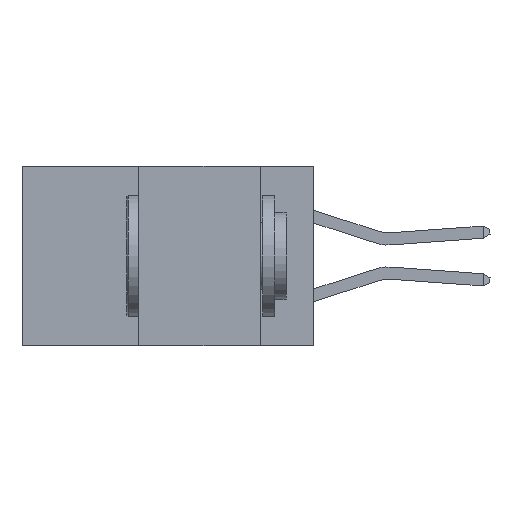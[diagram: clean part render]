
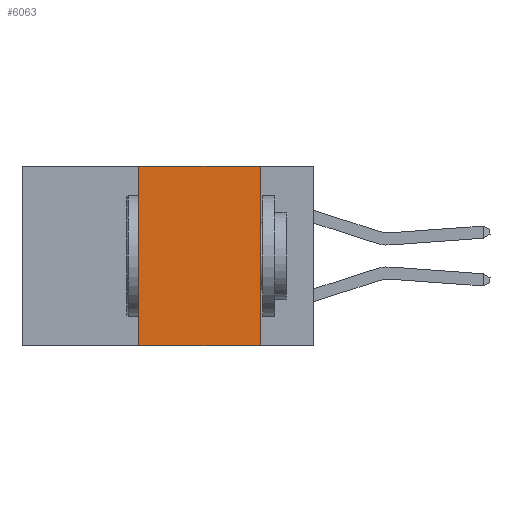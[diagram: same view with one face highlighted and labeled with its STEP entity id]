
A CAD part, left-side view. The second image highlights one B-rep face of the part: STEP entity #6063.
In plain terms, the highlighted planar face has unit normal (-1, 0, 0).
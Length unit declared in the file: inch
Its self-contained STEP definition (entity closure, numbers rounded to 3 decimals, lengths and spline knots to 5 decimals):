
#858 = AXIS2_PLACEMENT_3D ( 'NONE', #20803, #15157, #6983 ) ;
#1157 = VECTOR ( 'NONE', #2680, 39.37008 ) ;
#2680 = DIRECTION ( 'NONE',  ( 0., -1., 0. ) ) ;
#4364 = EDGE_CURVE ( 'NONE', #21309, #8622, #9887, .T. ) ;
#4973 = EDGE_LOOP ( 'NONE', ( #7449, #23508, #30149, #10833 ) ) ;
#5776 = VECTOR ( 'NONE', #22910, 39.37008 ) ;
#6063 = ADVANCED_FACE ( 'NONE', ( #34013 ), #12747, .F. ) ;
#6983 = DIRECTION ( 'NONE',  ( 0., 0., -1. ) ) ;
#6994 = VERTEX_POINT ( 'NONE', #29694 ) ;
#7449 = ORIENTED_EDGE ( 'NONE', *, *, #15761, .F. ) ;
#8044 = EDGE_CURVE ( 'NONE', #6994, #9968, #10895, .T. ) ;
#8622 = VERTEX_POINT ( 'NONE', #16449 ) ;
#9887 = LINE ( 'NONE', #34178, #32838 ) ;
#9968 = VERTEX_POINT ( 'NONE', #29895 ) ;
#10833 = ORIENTED_EDGE ( 'NONE', *, *, #8044, .T. ) ;
#10847 = DIRECTION ( 'NONE',  ( 0., 0., -1. ) ) ;
#10895 = LINE ( 'NONE', #16295, #1157 ) ;
#11619 = CARTESIAN_POINT ( 'NONE',  ( 0., 0.36, 0. ) ) ;
#12086 = LINE ( 'NONE', #20289, #5776 ) ;
#12123 = LINE ( 'NONE', #16080, #15553 ) ;
#12747 = PLANE ( 'NONE',  #858 ) ;
#15157 = DIRECTION ( 'NONE',  ( 1., 0., 0. ) ) ;
#15553 = VECTOR ( 'NONE', #10847, 39.37008 ) ;
#15761 = EDGE_CURVE ( 'NONE', #8622, #9968, #12123, .T. ) ;
#16080 = CARTESIAN_POINT ( 'NONE',  ( 0., 0.11, 0. ) ) ;
#16295 = CARTESIAN_POINT ( 'NONE',  ( 0., 0.6, -0.37 ) ) ;
#16449 = CARTESIAN_POINT ( 'NONE',  ( 0., 0.11, 0. ) ) ;
#20289 = CARTESIAN_POINT ( 'NONE',  ( 0., 0.36, 0. ) ) ;
#20803 = CARTESIAN_POINT ( 'NONE',  ( 0., 0.6, 0. ) ) ;
#21309 = VERTEX_POINT ( 'NONE', #11619 ) ;
#22910 = DIRECTION ( 'NONE',  ( 0., 0., 1. ) ) ;
#23508 = ORIENTED_EDGE ( 'NONE', *, *, #4364, .F. ) ;
#25860 = DIRECTION ( 'NONE',  ( 0., -1., 0. ) ) ;
#29694 = CARTESIAN_POINT ( 'NONE',  ( 0., 0.36, -0.37 ) ) ;
#29895 = CARTESIAN_POINT ( 'NONE',  ( 0., 0.11, -0.37 ) ) ;
#30149 = ORIENTED_EDGE ( 'NONE', *, *, #30311, .F. ) ;
#30311 = EDGE_CURVE ( 'NONE', #6994, #21309, #12086, .T. ) ;
#32838 = VECTOR ( 'NONE', #25860, 39.37008 ) ;
#34013 = FACE_OUTER_BOUND ( 'NONE', #4973, .T. ) ;
#34178 = CARTESIAN_POINT ( 'NONE',  ( 0., 0.6, 0. ) ) ;
